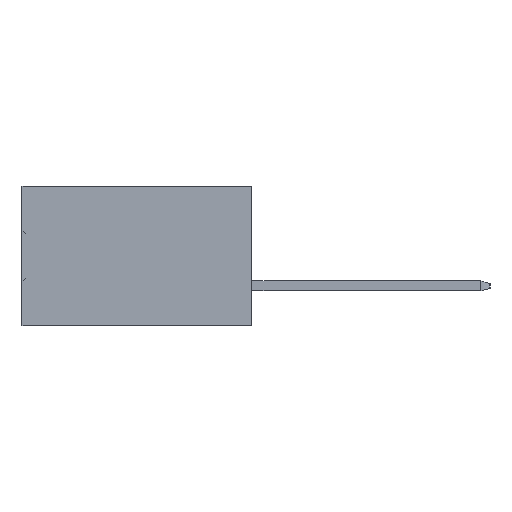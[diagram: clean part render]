
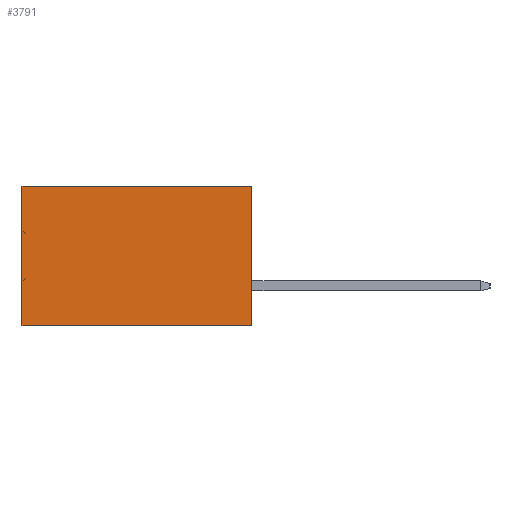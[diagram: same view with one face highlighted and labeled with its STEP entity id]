
A CAD part, left-side view. The second image highlights one B-rep face of the part: STEP entity #3791.
In plain terms, the highlighted planar face has unit normal (-1, 0, 0).
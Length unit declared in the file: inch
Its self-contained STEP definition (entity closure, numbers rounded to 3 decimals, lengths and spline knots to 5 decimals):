
#440 = EDGE_CURVE ( 'NONE', #11818, #6062, #4195, .T. ) ;
#1360 = AXIS2_PLACEMENT_3D ( 'NONE', #5812, #13101, #5972 ) ;
#1496 = LINE ( 'NONE', #10835, #26382 ) ;
#1665 = EDGE_CURVE ( 'NONE', #15115, #11818, #14998, .T. ) ;
#3791 = ADVANCED_FACE ( 'NONE', ( #6127 ), #22904, .F. ) ;
#4032 = DIRECTION ( 'NONE',  ( 0., 1., 0. ) ) ;
#4195 = LINE ( 'NONE', #28232, #20935 ) ;
#5812 = CARTESIAN_POINT ( 'NONE',  ( 0.3205, 0., -0.437 ) ) ;
#5972 = DIRECTION ( 'NONE',  ( 0., 0., -1. ) ) ;
#6062 = VERTEX_POINT ( 'NONE', #7121 ) ;
#6127 = FACE_OUTER_BOUND ( 'NONE', #11126, .T. ) ;
#6394 = DIRECTION ( 'NONE',  ( 0., 1., 0. ) ) ;
#7080 = DIRECTION ( 'NONE',  ( 0., 0., -1. ) ) ;
#7121 = CARTESIAN_POINT ( 'NONE',  ( 0.3205, 0.72, -0.437 ) ) ;
#7710 = CARTESIAN_POINT ( 'NONE',  ( 0.3205, 0.72, 0. ) ) ;
#8843 = VECTOR ( 'NONE', #24474, 39.37008 ) ;
#9051 = CARTESIAN_POINT ( 'NONE',  ( 0.3205, 0., 0. ) ) ;
#9599 = CARTESIAN_POINT ( 'NONE',  ( 0.3205, 0.72, -0.437 ) ) ;
#10617 = ORIENTED_EDGE ( 'NONE', *, *, #1665, .F. ) ;
#10835 = CARTESIAN_POINT ( 'NONE',  ( 0.3205, 0., 0. ) ) ;
#11126 = EDGE_LOOP ( 'NONE', ( #13249, #27663, #10617, #14629 ) ) ;
#11818 = VERTEX_POINT ( 'NONE', #13667 ) ;
#12868 = VECTOR ( 'NONE', #7080, 39.37008 ) ;
#13101 = DIRECTION ( 'NONE',  ( 1., 0., 0. ) ) ;
#13249 = ORIENTED_EDGE ( 'NONE', *, *, #22860, .T. ) ;
#13667 = CARTESIAN_POINT ( 'NONE',  ( 0.3205, 0., -0.437 ) ) ;
#14629 = ORIENTED_EDGE ( 'NONE', *, *, #17963, .T. ) ;
#14998 = LINE ( 'NONE', #17686, #8843 ) ;
#15115 = VERTEX_POINT ( 'NONE', #9051 ) ;
#17686 = CARTESIAN_POINT ( 'NONE',  ( 0.3205, 0., -0.437 ) ) ;
#17963 = EDGE_CURVE ( 'NONE', #15115, #18452, #1496, .T. ) ;
#18452 = VERTEX_POINT ( 'NONE', #7710 ) ;
#20935 = VECTOR ( 'NONE', #4032, 39.37008 ) ;
#22860 = EDGE_CURVE ( 'NONE', #18452, #6062, #28748, .T. ) ;
#22904 = PLANE ( 'NONE',  #1360 ) ;
#24474 = DIRECTION ( 'NONE',  ( 0., 0., -1. ) ) ;
#26382 = VECTOR ( 'NONE', #6394, 39.37008 ) ;
#27663 = ORIENTED_EDGE ( 'NONE', *, *, #440, .F. ) ;
#28232 = CARTESIAN_POINT ( 'NONE',  ( 0.3205, 0., -0.437 ) ) ;
#28748 = LINE ( 'NONE', #9599, #12868 ) ;
